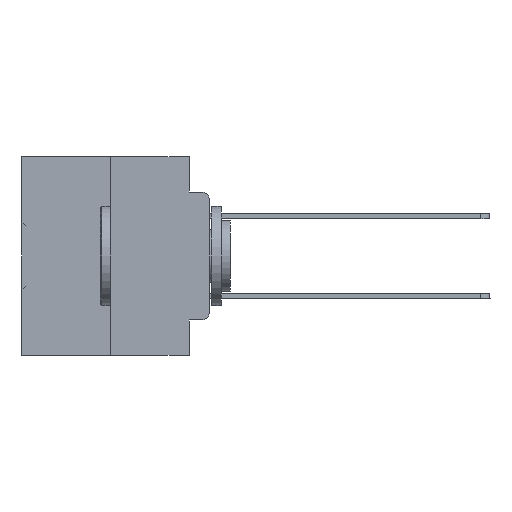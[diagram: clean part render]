
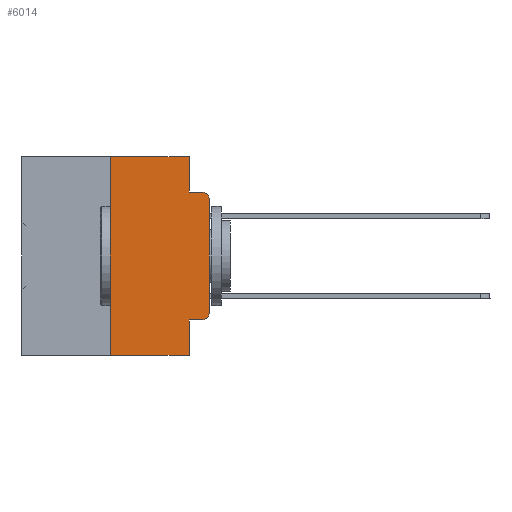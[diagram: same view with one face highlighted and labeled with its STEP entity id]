
A CAD part, left-side view. The second image highlights one B-rep face of the part: STEP entity #6014.
In plain terms, the highlighted planar face has unit normal (-1, 0, 0).
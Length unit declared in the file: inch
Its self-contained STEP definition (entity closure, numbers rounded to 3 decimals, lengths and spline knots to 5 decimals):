
#591 = ORIENTED_EDGE ( 'NONE', *, *, #21086, .F. ) ;
#666 = DIRECTION ( 'NONE',  ( -1., 0., 0. ) ) ;
#841 = LINE ( 'NONE', #7004, #29633 ) ;
#1666 = VERTEX_POINT ( 'NONE', #27434 ) ;
#2328 = CARTESIAN_POINT ( 'NONE',  ( 0., 0.473, -0.5 ) ) ;
#2395 = AXIS2_PLACEMENT_3D ( 'NONE', #15202, #11518, #22886 ) ;
#2428 = DIRECTION ( 'NONE',  ( 0., 0., -1. ) ) ;
#3272 = VERTEX_POINT ( 'NONE', #5339 ) ;
#3582 = EDGE_CURVE ( 'NONE', #8614, #19204, #841, .T. ) ;
#3764 = ORIENTED_EDGE ( 'NONE', *, *, #16437, .T. ) ;
#4027 = VERTEX_POINT ( 'NONE', #4476 ) ;
#4122 = LINE ( 'NONE', #27593, #28743 ) ;
#4476 = CARTESIAN_POINT ( 'NONE',  ( 0., 0., -0.1085 ) ) ;
#4558 = VERTEX_POINT ( 'NONE', #33524 ) ;
#4760 = EDGE_CURVE ( 'NONE', #11687, #1666, #17224, .T. ) ;
#5339 = CARTESIAN_POINT ( 'NONE',  ( 0., 0.25, 0. ) ) ;
#6014 = ADVANCED_FACE ( 'NONE', ( #15027 ), #28673, .F. ) ;
#7004 = CARTESIAN_POINT ( 'NONE',  ( 0., 0.051, -0.0885 ) ) ;
#8288 = DIRECTION ( 'NONE',  ( 0., -1., 0. ) ) ;
#8319 = CARTESIAN_POINT ( 'NONE',  ( 0., 0.051, -0.4115 ) ) ;
#8478 = VECTOR ( 'NONE', #24990, 39.37008 ) ;
#8614 = VERTEX_POINT ( 'NONE', #18220 ) ;
#8711 = ORIENTED_EDGE ( 'NONE', *, *, #34491, .T. ) ;
#9073 = ORIENTED_EDGE ( 'NONE', *, *, #28877, .F. ) ;
#10648 = DIRECTION ( 'NONE',  ( -1., 0., 0. ) ) ;
#11340 = CARTESIAN_POINT ( 'NONE',  ( 0., 0., 0. ) ) ;
#11465 = ORIENTED_EDGE ( 'NONE', *, *, #24324, .T. ) ;
#11518 = DIRECTION ( 'NONE',  ( 1., 0., 0. ) ) ;
#11687 = VERTEX_POINT ( 'NONE', #32654 ) ;
#12155 = CARTESIAN_POINT ( 'NONE',  ( 0., 0.051, -0.4115 ) ) ;
#12237 = DIRECTION ( 'NONE',  ( 0., -1., 0. ) ) ;
#12377 = VECTOR ( 'NONE', #25500, 39.37008 ) ;
#13035 = ORIENTED_EDGE ( 'NONE', *, *, #3582, .F. ) ;
#13403 = ORIENTED_EDGE ( 'NONE', *, *, #4760, .T. ) ;
#13435 = DIRECTION ( 'NONE',  ( 0., 0., -1. ) ) ;
#14119 = CARTESIAN_POINT ( 'NONE',  ( 0., 0.25, 0. ) ) ;
#15027 = FACE_OUTER_BOUND ( 'NONE', #24936, .T. ) ;
#15202 = CARTESIAN_POINT ( 'NONE',  ( 0., 0.473, 0. ) ) ;
#16051 = LINE ( 'NONE', #35851, #8478 ) ;
#16437 = EDGE_CURVE ( 'NONE', #1666, #4027, #28107, .T. ) ;
#17224 = CIRCLE ( 'NONE', #32733, 0.02 ) ;
#18220 = CARTESIAN_POINT ( 'NONE',  ( 0., 0.051, -0.0885 ) ) ;
#19204 = VERTEX_POINT ( 'NONE', #31782 ) ;
#19710 = DIRECTION ( 'NONE',  ( 0., -1., 0. ) ) ;
#20336 = CARTESIAN_POINT ( 'NONE',  ( 0., 0.051, 0. ) ) ;
#21086 = EDGE_CURVE ( 'NONE', #35883, #24898, #4122, .T. ) ;
#22886 = DIRECTION ( 'NONE',  ( 0., 0., -1. ) ) ;
#24231 = VERTEX_POINT ( 'NONE', #24513 ) ;
#24324 = EDGE_CURVE ( 'NONE', #4558, #24898, #33852, .T. ) ;
#24513 = CARTESIAN_POINT ( 'NONE',  ( 0., 0.051, 0. ) ) ;
#24631 = ORIENTED_EDGE ( 'NONE', *, *, #24695, .F. ) ;
#24665 = VECTOR ( 'NONE', #34322, 39.37008 ) ;
#24695 = EDGE_CURVE ( 'NONE', #24231, #8614, #34504, .T. ) ;
#24804 = VECTOR ( 'NONE', #19710, 39.37008 ) ;
#24898 = VERTEX_POINT ( 'NONE', #35050 ) ;
#24936 = EDGE_LOOP ( 'NONE', ( #3764, #8711, #13035, #24631, #9073, #30289, #11465, #591, #26028, #13403 ) ) ;
#24990 = DIRECTION ( 'NONE',  ( 0., -1., 0. ) ) ;
#25228 = EDGE_CURVE ( 'NONE', #4558, #3272, #31480, .T. ) ;
#25500 = DIRECTION ( 'NONE',  ( 0., 0., 1. ) ) ;
#26028 = ORIENTED_EDGE ( 'NONE', *, *, #36459, .T. ) ;
#27434 = CARTESIAN_POINT ( 'NONE',  ( 0., 0., -0.3915 ) ) ;
#27593 = CARTESIAN_POINT ( 'NONE',  ( 0., 0.051, 0. ) ) ;
#27626 = VECTOR ( 'NONE', #8288, 39.37008 ) ;
#27771 = AXIS2_PLACEMENT_3D ( 'NONE', #36204, #10648, #2428 ) ;
#28107 = LINE ( 'NONE', #11340, #12377 ) ;
#28673 = PLANE ( 'NONE',  #2395 ) ;
#28743 = VECTOR ( 'NONE', #13435, 39.37008 ) ;
#28877 = EDGE_CURVE ( 'NONE', #3272, #24231, #16051, .T. ) ;
#28891 = VECTOR ( 'NONE', #36518, 39.37008 ) ;
#29203 = DIRECTION ( 'NONE',  ( 0., 0., -1. ) ) ;
#29633 = VECTOR ( 'NONE', #12237, 39.37008 ) ;
#30289 = ORIENTED_EDGE ( 'NONE', *, *, #25228, .F. ) ;
#31480 = LINE ( 'NONE', #14119, #28891 ) ;
#31782 = CARTESIAN_POINT ( 'NONE',  ( 0., 0.02, -0.0885 ) ) ;
#31977 = CIRCLE ( 'NONE', #27771, 0.02 ) ;
#32654 = CARTESIAN_POINT ( 'NONE',  ( 0., 0.02, -0.4115 ) ) ;
#32733 = AXIS2_PLACEMENT_3D ( 'NONE', #34450, #666, #29203 ) ;
#33524 = CARTESIAN_POINT ( 'NONE',  ( 0., 0.25, -0.5 ) ) ;
#33852 = LINE ( 'NONE', #2328, #27626 ) ;
#34322 = DIRECTION ( 'NONE',  ( 0., 0., -1. ) ) ;
#34450 = CARTESIAN_POINT ( 'NONE',  ( 0., 0.02, -0.3915 ) ) ;
#34491 = EDGE_CURVE ( 'NONE', #4027, #19204, #31977, .T. ) ;
#34504 = LINE ( 'NONE', #20336, #24665 ) ;
#35050 = CARTESIAN_POINT ( 'NONE',  ( 0., 0.051, -0.5 ) ) ;
#35851 = CARTESIAN_POINT ( 'NONE',  ( 0., 0.473, 0. ) ) ;
#35883 = VERTEX_POINT ( 'NONE', #12155 ) ;
#36204 = CARTESIAN_POINT ( 'NONE',  ( 0., 0.02, -0.1085 ) ) ;
#36459 = EDGE_CURVE ( 'NONE', #35883, #11687, #36698, .T. ) ;
#36518 = DIRECTION ( 'NONE',  ( 0., 0., 1. ) ) ;
#36698 = LINE ( 'NONE', #8319, #24804 ) ;
